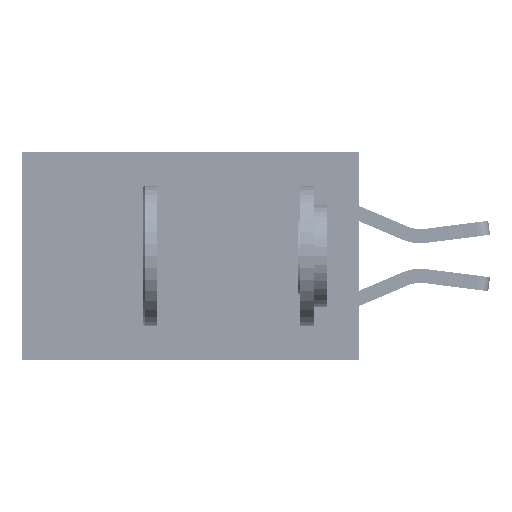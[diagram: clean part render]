
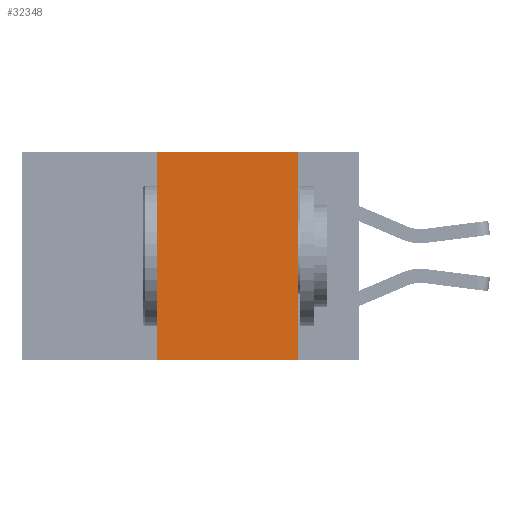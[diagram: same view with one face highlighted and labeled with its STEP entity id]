
A CAD part, left-side view. The second image highlights one B-rep face of the part: STEP entity #32348.
In plain terms, the highlighted planar face has unit normal (-1, 0, 0).
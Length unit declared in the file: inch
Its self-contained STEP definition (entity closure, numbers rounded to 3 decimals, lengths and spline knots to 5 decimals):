
#1554 = CARTESIAN_POINT ( 'NONE',  ( 0., 0.6, 0. ) ) ;
#1717 = DIRECTION ( 'NONE',  ( 1., 0., 0. ) ) ;
#1756 = EDGE_CURVE ( 'NONE', #31490, #14733, #28432, .T. ) ;
#3226 = EDGE_CURVE ( 'NONE', #5587, #31490, #21282, .T. ) ;
#3671 = AXIS2_PLACEMENT_3D ( 'NONE', #1554, #1717, #29801 ) ;
#4629 = CARTESIAN_POINT ( 'NONE',  ( 0., 0.36, 0. ) ) ;
#5050 = CARTESIAN_POINT ( 'NONE',  ( 0., 0.36, 0. ) ) ;
#5587 = VERTEX_POINT ( 'NONE', #38219 ) ;
#7304 = CARTESIAN_POINT ( 'NONE',  ( 0., 0.11, -0.37 ) ) ;
#8016 = ORIENTED_EDGE ( 'NONE', *, *, #1756, .F. ) ;
#8656 = CARTESIAN_POINT ( 'NONE',  ( 0., 0.11, 0. ) ) ;
#9608 = VERTEX_POINT ( 'NONE', #7304 ) ;
#10751 = DIRECTION ( 'NONE',  ( 0., -1., 0. ) ) ;
#11232 = FACE_OUTER_BOUND ( 'NONE', #19111, .T. ) ;
#13274 = ORIENTED_EDGE ( 'NONE', *, *, #3226, .F. ) ;
#13895 = PLANE ( 'NONE',  #3671 ) ;
#14733 = VERTEX_POINT ( 'NONE', #8656 ) ;
#19111 = EDGE_LOOP ( 'NONE', ( #37231, #8016, #13274, #34843 ) ) ;
#19901 = VECTOR ( 'NONE', #10751, 39.37008 ) ;
#21282 = LINE ( 'NONE', #5050, #32659 ) ;
#22175 = DIRECTION ( 'NONE',  ( 0., 0., -1. ) ) ;
#22215 = CARTESIAN_POINT ( 'NONE',  ( 0., 0.6, -0.37 ) ) ;
#24102 = VECTOR ( 'NONE', #22175, 39.37008 ) ;
#25728 = EDGE_CURVE ( 'NONE', #5587, #9608, #42709, .T. ) ;
#27895 = EDGE_CURVE ( 'NONE', #14733, #9608, #47481, .T. ) ;
#28432 = LINE ( 'NONE', #36847, #40499 ) ;
#29761 = DIRECTION ( 'NONE',  ( 0., 0., 1. ) ) ;
#29801 = DIRECTION ( 'NONE',  ( 0., 0., -1. ) ) ;
#31490 = VERTEX_POINT ( 'NONE', #4629 ) ;
#32348 = ADVANCED_FACE ( 'NONE', ( #11232 ), #13895, .F. ) ;
#32659 = VECTOR ( 'NONE', #29761, 39.37008 ) ;
#34211 = CARTESIAN_POINT ( 'NONE',  ( 0., 0.11, 0. ) ) ;
#34843 = ORIENTED_EDGE ( 'NONE', *, *, #25728, .T. ) ;
#36847 = CARTESIAN_POINT ( 'NONE',  ( 0., 0.6, 0. ) ) ;
#37231 = ORIENTED_EDGE ( 'NONE', *, *, #27895, .F. ) ;
#37562 = DIRECTION ( 'NONE',  ( 0., -1., 0. ) ) ;
#38219 = CARTESIAN_POINT ( 'NONE',  ( 0., 0.36, -0.37 ) ) ;
#40499 = VECTOR ( 'NONE', #37562, 39.37008 ) ;
#42709 = LINE ( 'NONE', #22215, #19901 ) ;
#47481 = LINE ( 'NONE', #34211, #24102 ) ;
